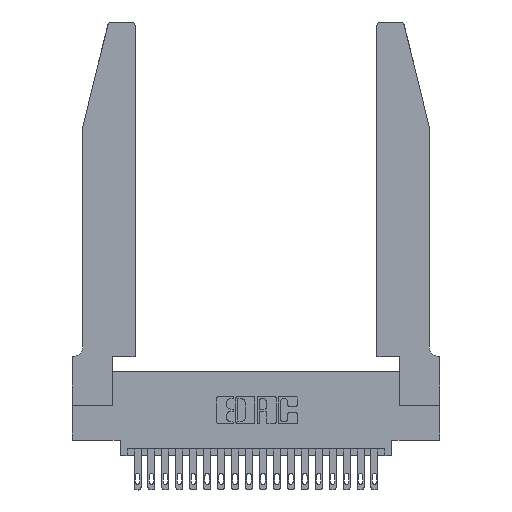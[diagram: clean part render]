
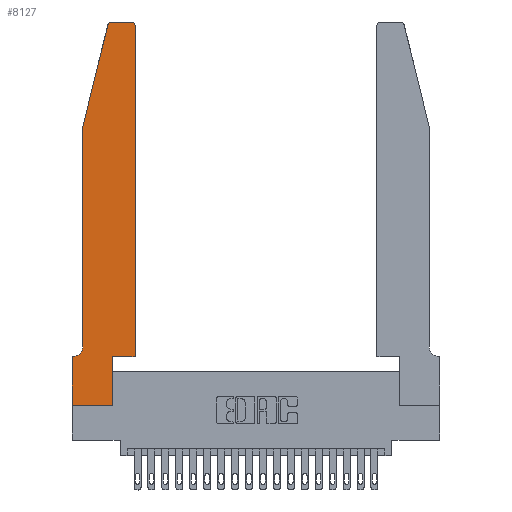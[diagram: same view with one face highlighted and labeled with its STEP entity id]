
A CAD part, top view. The second image highlights one B-rep face of the part: STEP entity #8127.
In plain terms, the highlighted planar face has unit normal (0, 0, 1).
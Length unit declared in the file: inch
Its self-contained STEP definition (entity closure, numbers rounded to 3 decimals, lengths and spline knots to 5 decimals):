
#846 = DIRECTION ( 'NONE',  ( 0., 0., 1. ) ) ;
#1418 = ORIENTED_EDGE ( 'NONE', *, *, #16580, .T. ) ;
#2150 = LINE ( 'NONE', #3093, #5347 ) ;
#2698 = VERTEX_POINT ( 'NONE', #7408 ) ;
#2732 = VERTEX_POINT ( 'NONE', #21996 ) ;
#2876 = VECTOR ( 'NONE', #3306, 39.37008 ) ;
#3093 = CARTESIAN_POINT ( 'NONE',  ( 0.4505, 0.35, 0.37 ) ) ;
#3262 = CARTESIAN_POINT ( 'NONE',  ( 0.2865, 0.35, 0.37 ) ) ;
#3306 = DIRECTION ( 'NONE',  ( -1., 0., 0. ) ) ;
#3702 = CARTESIAN_POINT ( 'NONE',  ( 0.0055, 0.42, 0.37 ) ) ;
#3747 = EDGE_CURVE ( 'NONE', #2698, #6375, #17826, .T. ) ;
#3886 = CARTESIAN_POINT ( 'NONE',  ( 0.4505, 0.35, 0.37 ) ) ;
#3929 = CARTESIAN_POINT ( 'NONE',  ( 0.25487, 2.72718, 0.37 ) ) ;
#4511 = CARTESIAN_POINT ( 'NONE',  ( 0., 0., 0.37 ) ) ;
#4538 = VERTEX_POINT ( 'NONE', #3886 ) ;
#4728 = CIRCLE ( 'NONE', #17908, 0.07 ) ;
#4854 = LINE ( 'NONE', #20087, #18523 ) ;
#5347 = VECTOR ( 'NONE', #15703, 39.37008 ) ;
#5356 = ORIENTED_EDGE ( 'NONE', *, *, #7073, .T. ) ;
#5872 = ORIENTED_EDGE ( 'NONE', *, *, #20410, .T. ) ;
#5895 = VECTOR ( 'NONE', #9190, 39.37008 ) ;
#6375 = VERTEX_POINT ( 'NONE', #3929 ) ;
#6381 = FACE_OUTER_BOUND ( 'NONE', #18317, .T. ) ;
#6556 = CARTESIAN_POINT ( 'NONE',  ( 0., 0., 0.37 ) ) ;
#6745 = DIRECTION ( 'NONE',  ( 1., 0., 0. ) ) ;
#7029 = PLANE ( 'NONE',  #8264 ) ;
#7073 = EDGE_CURVE ( 'NONE', #4538, #9103, #2150, .T. ) ;
#7402 = CARTESIAN_POINT ( 'NONE',  ( 0., 0., 0.37 ) ) ;
#7408 = CARTESIAN_POINT ( 'NONE',  ( 0.284, 2.75, 0.37 ) ) ;
#7678 = LINE ( 'NONE', #15029, #2876 ) ;
#7902 = CARTESIAN_POINT ( 'NONE',  ( 0.2605, 2.75, 0.37 ) ) ;
#8127 = ADVANCED_FACE ( 'NONE', ( #6381 ), #7029, .T. ) ;
#8264 = AXIS2_PLACEMENT_3D ( 'NONE', #19013, #18878, #17367 ) ;
#8581 = VERTEX_POINT ( 'NONE', #19620 ) ;
#8612 = EDGE_CURVE ( 'NONE', #14683, #8581, #4728, .T. ) ;
#8641 = LINE ( 'NONE', #6556, #11044 ) ;
#8874 = CARTESIAN_POINT ( 'NONE',  ( 0.0755, 2., 0.37 ) ) ;
#9103 = VERTEX_POINT ( 'NONE', #14882 ) ;
#9163 = EDGE_CURVE ( 'NONE', #8581, #13646, #7678, .T. ) ;
#9190 = DIRECTION ( 'NONE',  ( -0.239, -0.971, 0. ) ) ;
#9362 = CARTESIAN_POINT ( 'NONE',  ( 0.284, 2.72, 0.37 ) ) ;
#9938 = VERTEX_POINT ( 'NONE', #10351 ) ;
#10020 = ORIENTED_EDGE ( 'NONE', *, *, #9163, .T. ) ;
#10148 = DIRECTION ( 'NONE',  ( 1., 0., 0. ) ) ;
#10309 = AXIS2_PLACEMENT_3D ( 'NONE', #18676, #20404, #10148 ) ;
#10351 = CARTESIAN_POINT ( 'NONE',  ( 0.0755, 2., 0.37 ) ) ;
#11044 = VECTOR ( 'NONE', #16667, 39.37008 ) ;
#11415 = EDGE_CURVE ( 'NONE', #9938, #14683, #19259, .T. ) ;
#11484 = DIRECTION ( 'NONE',  ( -1., 0., 0. ) ) ;
#11744 = VERTEX_POINT ( 'NONE', #4511 ) ;
#12004 = DIRECTION ( 'NONE',  ( 0., 1., 0. ) ) ;
#12010 = ORIENTED_EDGE ( 'NONE', *, *, #3747, .T. ) ;
#12289 = DIRECTION ( 'NONE',  ( -1., 0., 0. ) ) ;
#12983 = CARTESIAN_POINT ( 'NONE',  ( 0.2865, 0., 0.37 ) ) ;
#13152 = VECTOR ( 'NONE', #19703, 39.37008 ) ;
#13617 = ORIENTED_EDGE ( 'NONE', *, *, #11415, .T. ) ;
#13646 = VERTEX_POINT ( 'NONE', #18650 ) ;
#14109 = VERTEX_POINT ( 'NONE', #12983 ) ;
#14145 = ORIENTED_EDGE ( 'NONE', *, *, #14899, .T. ) ;
#14287 = CARTESIAN_POINT ( 'NONE',  ( 0.4205, 2.75, 0.37 ) ) ;
#14378 = ORIENTED_EDGE ( 'NONE', *, *, #19203, .T. ) ;
#14508 = DIRECTION ( 'NONE',  ( 1., 0., 0. ) ) ;
#14683 = VERTEX_POINT ( 'NONE', #18006 ) ;
#14882 = CARTESIAN_POINT ( 'NONE',  ( 0.4505, 2.72, 0.37 ) ) ;
#14899 = EDGE_CURVE ( 'NONE', #14109, #2732, #20749, .T. ) ;
#15029 = CARTESIAN_POINT ( 'NONE',  ( 0.0755, 0.35, 0.37 ) ) ;
#15248 = LINE ( 'NONE', #7902, #16594 ) ;
#15703 = DIRECTION ( 'NONE',  ( 0., 1., 0. ) ) ;
#15839 = ORIENTED_EDGE ( 'NONE', *, *, #19522, .T. ) ;
#16000 = EDGE_CURVE ( 'NONE', #13646, #11744, #8641, .T. ) ;
#16108 = CIRCLE ( 'NONE', #10309, 0.03 ) ;
#16550 = ORIENTED_EDGE ( 'NONE', *, *, #8612, .T. ) ;
#16580 = EDGE_CURVE ( 'NONE', #6375, #9938, #18876, .T. ) ;
#16594 = VECTOR ( 'NONE', #11484, 39.37008 ) ;
#16667 = DIRECTION ( 'NONE',  ( 0., -1., 0. ) ) ;
#16978 = AXIS2_PLACEMENT_3D ( 'NONE', #9362, #846, #14508 ) ;
#17367 = DIRECTION ( 'NONE',  ( 1., 0., 0. ) ) ;
#17393 = DIRECTION ( 'NONE',  ( 0., 0., -1. ) ) ;
#17727 = LINE ( 'NONE', #7402, #13152 ) ;
#17826 = CIRCLE ( 'NONE', #16978, 0.03 ) ;
#17908 = AXIS2_PLACEMENT_3D ( 'NONE', #3702, #17393, #12289 ) ;
#18006 = CARTESIAN_POINT ( 'NONE',  ( 0.0755, 0.42, 0.37 ) ) ;
#18317 = EDGE_LOOP ( 'NONE', ( #5872, #12010, #1418, #13617, #16550, #10020, #21512, #15839, #14145, #14378, #5356, #19661 ) ) ;
#18523 = VECTOR ( 'NONE', #6745, 39.37008 ) ;
#18650 = CARTESIAN_POINT ( 'NONE',  ( 0., 0.35, 0.37 ) ) ;
#18669 = EDGE_CURVE ( 'NONE', #9103, #21588, #16108, .T. ) ;
#18676 = CARTESIAN_POINT ( 'NONE',  ( 0.4205, 2.72, 0.37 ) ) ;
#18876 = LINE ( 'NONE', #8874, #5895 ) ;
#18878 = DIRECTION ( 'NONE',  ( 0., 0., 1. ) ) ;
#18987 = VECTOR ( 'NONE', #20398, 39.37008 ) ;
#19013 = CARTESIAN_POINT ( 'NONE',  ( 0., 0.35, 0.37 ) ) ;
#19203 = EDGE_CURVE ( 'NONE', #2732, #4538, #4854, .T. ) ;
#19259 = LINE ( 'NONE', #20625, #18987 ) ;
#19522 = EDGE_CURVE ( 'NONE', #11744, #14109, #17727, .T. ) ;
#19620 = CARTESIAN_POINT ( 'NONE',  ( 0.0055, 0.35, 0.37 ) ) ;
#19661 = ORIENTED_EDGE ( 'NONE', *, *, #18669, .T. ) ;
#19703 = DIRECTION ( 'NONE',  ( 1., 0., 0. ) ) ;
#20087 = CARTESIAN_POINT ( 'NONE',  ( 0.4505, 0.35, 0.37 ) ) ;
#20398 = DIRECTION ( 'NONE',  ( 0., -1., 0. ) ) ;
#20404 = DIRECTION ( 'NONE',  ( 0., 0., 1. ) ) ;
#20410 = EDGE_CURVE ( 'NONE', #21588, #2698, #15248, .T. ) ;
#20625 = CARTESIAN_POINT ( 'NONE',  ( 0.0755, 2., 0.37 ) ) ;
#20749 = LINE ( 'NONE', #3262, #22120 ) ;
#21512 = ORIENTED_EDGE ( 'NONE', *, *, #16000, .T. ) ;
#21588 = VERTEX_POINT ( 'NONE', #14287 ) ;
#21996 = CARTESIAN_POINT ( 'NONE',  ( 0.2865, 0.35, 0.37 ) ) ;
#22120 = VECTOR ( 'NONE', #12004, 39.37008 ) ;
